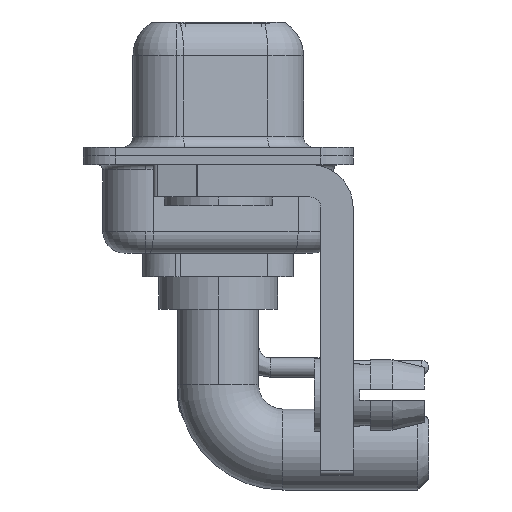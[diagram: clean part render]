
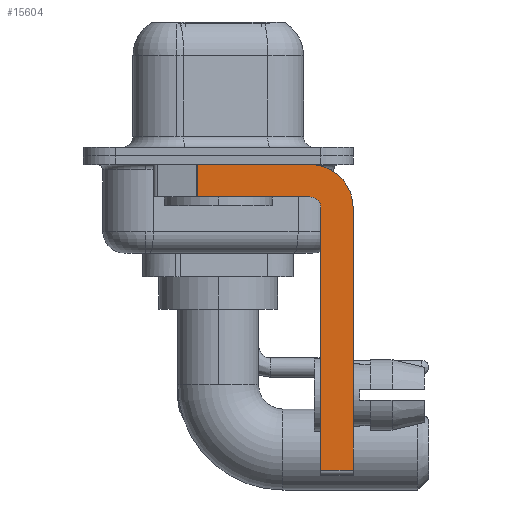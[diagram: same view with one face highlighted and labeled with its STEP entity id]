
A CAD part, left-side view. The second image highlights one B-rep face of the part: STEP entity #15604.
In plain terms, the highlighted planar face has unit normal (-1, 0, 0).
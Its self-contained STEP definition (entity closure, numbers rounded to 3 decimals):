
#114 = EDGE_CURVE ( 'NONE', #21372, #1618, #9137, .T. ) ;
#205 = CARTESIAN_POINT ( 'NONE',  ( -2.9, 0.978, -1.9 ) ) ;
#1551 = EDGE_CURVE ( 'NONE', #16052, #21372, #21090, .T. ) ;
#1618 = VERTEX_POINT ( 'NONE', #16275 ) ;
#1655 = EDGE_CURVE ( 'NONE', #9287, #15771, #18908, .T. ) ;
#2477 = CARTESIAN_POINT ( 'NONE',  ( -2.9, -4.25, -1.9 ) ) ;
#2480 = DIRECTION ( 'NONE',  ( 0., 0., -1. ) ) ;
#2891 = DIRECTION ( 'NONE',  ( 0., -1., 0. ) ) ;
#2915 = DIRECTION ( 'NONE',  ( 0., -1., 0. ) ) ;
#3147 = VECTOR ( 'NONE', #2891, 1000. ) ;
#3517 = CARTESIAN_POINT ( 'NONE',  ( -2.9, 0.978, -0.4 ) ) ;
#3547 = PLANE ( 'NONE',  #5959 ) ;
#3621 = ORIENTED_EDGE ( 'NONE', *, *, #13883, .T. ) ;
#3828 = CARTESIAN_POINT ( 'NONE',  ( -2.9, -4.25, -1.9 ) ) ;
#3869 = VECTOR ( 'NONE', #14505, 1000. ) ;
#4132 = VECTOR ( 'NONE', #22995, 1000. ) ;
#4651 = CARTESIAN_POINT ( 'NONE',  ( -2.9, 3., -0.4 ) ) ;
#5235 = CARTESIAN_POINT ( 'NONE',  ( -2.9, -4.25, -2.4 ) ) ;
#5600 = VECTOR ( 'NONE', #2915, 1000. ) ;
#5959 = AXIS2_PLACEMENT_3D ( 'NONE', #7069, #10824, #21850 ) ;
#6464 = CARTESIAN_POINT ( 'NONE',  ( -2.9, -4.25, -2.4 ) ) ;
#6875 = CARTESIAN_POINT ( 'NONE',  ( -2.9, -6.25, -14.55 ) ) ;
#7069 = CARTESIAN_POINT ( 'NONE',  ( -2.9, -4.25, -2.4 ) ) ;
#7106 = CARTESIAN_POINT ( 'NONE',  ( -2.9, -4.25, -14.55 ) ) ;
#8984 = CARTESIAN_POINT ( 'NONE',  ( -2.9, 0.978, -1.9 ) ) ;
#9137 = CIRCLE ( 'NONE', #17033, 2. ) ;
#9287 = VERTEX_POINT ( 'NONE', #15503 ) ;
#9492 = CARTESIAN_POINT ( 'NONE',  ( -2.9, -4.75, -14.55 ) ) ;
#10824 = DIRECTION ( 'NONE',  ( 1., 0., 0. ) ) ;
#10972 = DIRECTION ( 'NONE',  ( -1., 0., 0. ) ) ;
#11524 = DIRECTION ( 'NONE',  ( 1., 0., 0. ) ) ;
#11638 = VECTOR ( 'NONE', #16404, 1000. ) ;
#12432 = LINE ( 'NONE', #19600, #4132 ) ;
#13883 = EDGE_CURVE ( 'NONE', #16052, #18282, #16263, .T. ) ;
#14033 = ORIENTED_EDGE ( 'NONE', *, *, #17360, .F. ) ;
#14464 = FACE_OUTER_BOUND ( 'NONE', #22366, .T. ) ;
#14505 = DIRECTION ( 'NONE',  ( 0., 1., 0. ) ) ;
#14619 = LINE ( 'NONE', #18168, #11638 ) ;
#14724 = LINE ( 'NONE', #3828, #3869 ) ;
#15247 = ORIENTED_EDGE ( 'NONE', *, *, #21427, .F. ) ;
#15503 = CARTESIAN_POINT ( 'NONE',  ( -2.9, -4.75, -2.4 ) ) ;
#15604 = ADVANCED_FACE ( 'NONE', ( #14464 ), #3547, .F. ) ;
#15771 = VERTEX_POINT ( 'NONE', #2477 ) ;
#16036 = LINE ( 'NONE', #7106, #5600 ) ;
#16052 = VERTEX_POINT ( 'NONE', #3517 ) ;
#16263 = LINE ( 'NONE', #8984, #21677 ) ;
#16275 = CARTESIAN_POINT ( 'NONE',  ( -2.9, -6.25, -2.4 ) ) ;
#16348 = EDGE_CURVE ( 'NONE', #18190, #21323, #16036, .T. ) ;
#16404 = DIRECTION ( 'NONE',  ( 0., 0., 1. ) ) ;
#16671 = AXIS2_PLACEMENT_3D ( 'NONE', #5235, #10972, #21209 ) ;
#17033 = AXIS2_PLACEMENT_3D ( 'NONE', #6464, #11524, #2480 ) ;
#17197 = EDGE_CURVE ( 'NONE', #1618, #21323, #12432, .T. ) ;
#17360 = EDGE_CURVE ( 'NONE', #18190, #9287, #14619, .T. ) ;
#18143 = DIRECTION ( 'NONE',  ( 0., 0., -1. ) ) ;
#18168 = CARTESIAN_POINT ( 'NONE',  ( -2.9, -4.75, -14.8 ) ) ;
#18190 = VERTEX_POINT ( 'NONE', #9492 ) ;
#18282 = VERTEX_POINT ( 'NONE', #205 ) ;
#18908 = CIRCLE ( 'NONE', #16671, 0.5 ) ;
#19385 = ORIENTED_EDGE ( 'NONE', *, *, #1551, .F. ) ;
#19600 = CARTESIAN_POINT ( 'NONE',  ( -2.9, -6.25, -2.4 ) ) ;
#19881 = ORIENTED_EDGE ( 'NONE', *, *, #1655, .F. ) ;
#21090 = LINE ( 'NONE', #4651, #3147 ) ;
#21209 = DIRECTION ( 'NONE',  ( 0., 0., 1. ) ) ;
#21323 = VERTEX_POINT ( 'NONE', #6875 ) ;
#21372 = VERTEX_POINT ( 'NONE', #21896 ) ;
#21427 = EDGE_CURVE ( 'NONE', #15771, #18282, #14724, .T. ) ;
#21677 = VECTOR ( 'NONE', #18143, 1000. ) ;
#21683 = ORIENTED_EDGE ( 'NONE', *, *, #114, .F. ) ;
#21818 = ORIENTED_EDGE ( 'NONE', *, *, #17197, .F. ) ;
#21850 = DIRECTION ( 'NONE',  ( 0., 0., -1. ) ) ;
#21896 = CARTESIAN_POINT ( 'NONE',  ( -2.9, -4.25, -0.4 ) ) ;
#22366 = EDGE_LOOP ( 'NONE', ( #19385, #3621, #15247, #19881, #14033, #22625, #21818, #21683 ) ) ;
#22625 = ORIENTED_EDGE ( 'NONE', *, *, #16348, .T. ) ;
#22995 = DIRECTION ( 'NONE',  ( 0., 0., -1. ) ) ;
